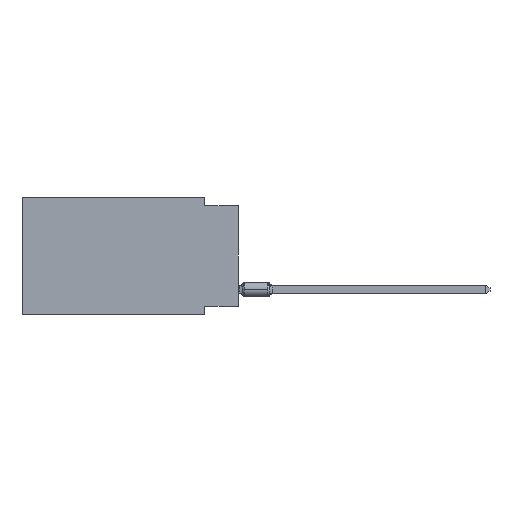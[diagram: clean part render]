
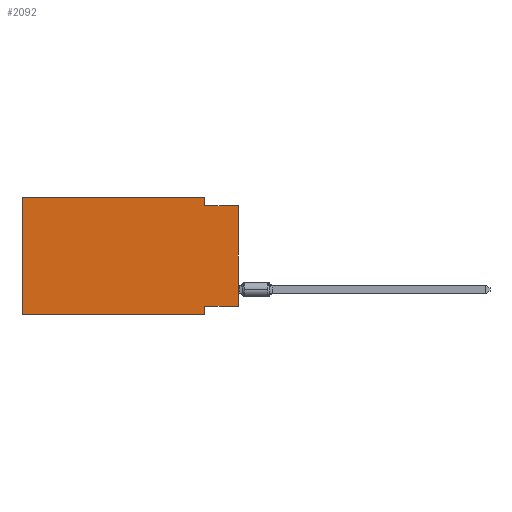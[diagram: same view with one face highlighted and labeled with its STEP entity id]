
A CAD part, left-side view. The second image highlights one B-rep face of the part: STEP entity #2092.
In plain terms, the highlighted planar face has unit normal (-1, 0, 0).
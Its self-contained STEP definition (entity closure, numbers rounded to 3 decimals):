
#589 = ORIENTED_EDGE ( 'NONE', *, *, #21772, .F. ) ;
#1047 = LINE ( 'NONE', #14686, #12461 ) ;
#1093 = DIRECTION ( 'NONE',  ( 0., 0., -1. ) ) ;
#1754 = CARTESIAN_POINT ( 'NONE',  ( 0., 16.383, 0. ) ) ;
#1766 = PLANE ( 'NONE',  #23817 ) ;
#1850 = CARTESIAN_POINT ( 'NONE',  ( 0., 2.54, 0. ) ) ;
#1980 = LINE ( 'NONE', #13682, #1992 ) ;
#1992 = VECTOR ( 'NONE', #13932, 1000. ) ;
#2092 = ADVANCED_FACE ( 'NONE', ( #21316 ), #1766, .F. ) ;
#2708 = VERTEX_POINT ( 'NONE', #18561 ) ;
#2920 = CARTESIAN_POINT ( 'NONE',  ( 0., 2.54, 0. ) ) ;
#3158 = EDGE_CURVE ( 'NONE', #17540, #6567, #22010, .T. ) ;
#3869 = EDGE_CURVE ( 'NONE', #6567, #9959, #1980, .T. ) ;
#4143 = VERTEX_POINT ( 'NONE', #13520 ) ;
#4228 = DIRECTION ( 'NONE',  ( 0., 0., -1. ) ) ;
#4587 = LINE ( 'NONE', #8450, #22129 ) ;
#4744 = ORIENTED_EDGE ( 'NONE', *, *, #3869, .F. ) ;
#4966 = VECTOR ( 'NONE', #7158, 1000. ) ;
#6064 = ORIENTED_EDGE ( 'NONE', *, *, #9190, .F. ) ;
#6098 = CARTESIAN_POINT ( 'NONE',  ( 0., 16.383, -8.89 ) ) ;
#6567 = VERTEX_POINT ( 'NONE', #1754 ) ;
#6846 = DIRECTION ( 'NONE',  ( 0., -1., 0. ) ) ;
#7033 = VERTEX_POINT ( 'NONE', #17676 ) ;
#7158 = DIRECTION ( 'NONE',  ( 0., 1., 0. ) ) ;
#8064 = CARTESIAN_POINT ( 'NONE',  ( 0., 2.54, -0.635 ) ) ;
#8151 = LINE ( 'NONE', #6098, #12840 ) ;
#8450 = CARTESIAN_POINT ( 'NONE',  ( 0., 2.54, -8.89 ) ) ;
#9190 = EDGE_CURVE ( 'NONE', #7033, #2708, #16955, .T. ) ;
#9959 = VERTEX_POINT ( 'NONE', #1850 ) ;
#10161 = CARTESIAN_POINT ( 'NONE',  ( 0., 16.383, -8.89 ) ) ;
#10218 = ORIENTED_EDGE ( 'NONE', *, *, #11162, .T. ) ;
#10809 = ORIENTED_EDGE ( 'NONE', *, *, #3158, .F. ) ;
#10968 = VERTEX_POINT ( 'NONE', #17473 ) ;
#11035 = ORIENTED_EDGE ( 'NONE', *, *, #14966, .F. ) ;
#11162 = EDGE_CURVE ( 'NONE', #17540, #10968, #8151, .T. ) ;
#11439 = ORIENTED_EDGE ( 'NONE', *, *, #20841, .T. ) ;
#12134 = DIRECTION ( 'NONE',  ( 0., -1., 0. ) ) ;
#12461 = VECTOR ( 'NONE', #22535, 1000. ) ;
#12648 = VECTOR ( 'NONE', #19955, 1000. ) ;
#12840 = VECTOR ( 'NONE', #12134, 1000. ) ;
#13341 = CARTESIAN_POINT ( 'NONE',  ( 0., 16.383, 0. ) ) ;
#13520 = CARTESIAN_POINT ( 'NONE',  ( 0., 0., -0.635 ) ) ;
#13682 = CARTESIAN_POINT ( 'NONE',  ( 0., 16.383, 0. ) ) ;
#13926 = VECTOR ( 'NONE', #1093, 1000. ) ;
#13932 = DIRECTION ( 'NONE',  ( 0., -1., 0. ) ) ;
#14686 = CARTESIAN_POINT ( 'NONE',  ( 0., 0., 0. ) ) ;
#14966 = EDGE_CURVE ( 'NONE', #2708, #10968, #4587, .T. ) ;
#15094 = EDGE_CURVE ( 'NONE', #9959, #21983, #18355, .T. ) ;
#15640 = ORIENTED_EDGE ( 'NONE', *, *, #15094, .F. ) ;
#16646 = LINE ( 'NONE', #24490, #24026 ) ;
#16955 = LINE ( 'NONE', #24807, #4966 ) ;
#17332 = DIRECTION ( 'NONE',  ( 0., 0., -1. ) ) ;
#17473 = CARTESIAN_POINT ( 'NONE',  ( 0., 2.54, -8.89 ) ) ;
#17540 = VERTEX_POINT ( 'NONE', #10161 ) ;
#17676 = CARTESIAN_POINT ( 'NONE',  ( 0., 0., -8.255 ) ) ;
#18037 = EDGE_LOOP ( 'NONE', ( #11439, #589, #15640, #4744, #10809, #10218, #11035, #6064 ) ) ;
#18355 = LINE ( 'NONE', #2920, #13926 ) ;
#18561 = CARTESIAN_POINT ( 'NONE',  ( 0., 2.54, -8.255 ) ) ;
#19394 = DIRECTION ( 'NONE',  ( 1., 0., 0. ) ) ;
#19955 = DIRECTION ( 'NONE',  ( 0., 0., 1. ) ) ;
#20841 = EDGE_CURVE ( 'NONE', #7033, #4143, #1047, .T. ) ;
#21316 = FACE_OUTER_BOUND ( 'NONE', #18037, .T. ) ;
#21772 = EDGE_CURVE ( 'NONE', #21983, #4143, #16646, .T. ) ;
#21898 = CARTESIAN_POINT ( 'NONE',  ( 0., 16.383, 0. ) ) ;
#21983 = VERTEX_POINT ( 'NONE', #8064 ) ;
#22010 = LINE ( 'NONE', #21898, #12648 ) ;
#22129 = VECTOR ( 'NONE', #4228, 1000. ) ;
#22535 = DIRECTION ( 'NONE',  ( 0., 0., 1. ) ) ;
#23817 = AXIS2_PLACEMENT_3D ( 'NONE', #13341, #19394, #17332 ) ;
#24026 = VECTOR ( 'NONE', #6846, 1000. ) ;
#24490 = CARTESIAN_POINT ( 'NONE',  ( 0., 0., -0.635 ) ) ;
#24807 = CARTESIAN_POINT ( 'NONE',  ( 0., 0., -8.255 ) ) ;
